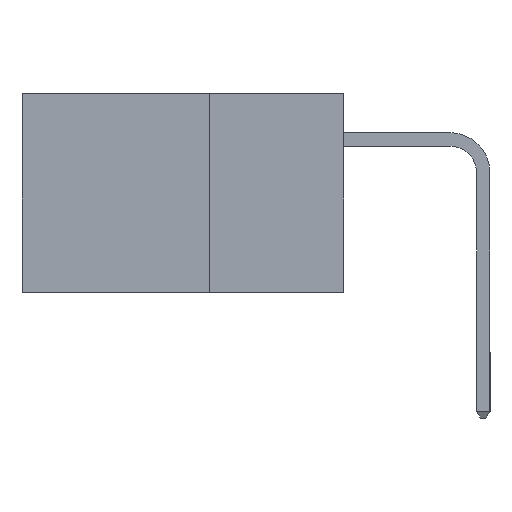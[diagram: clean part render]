
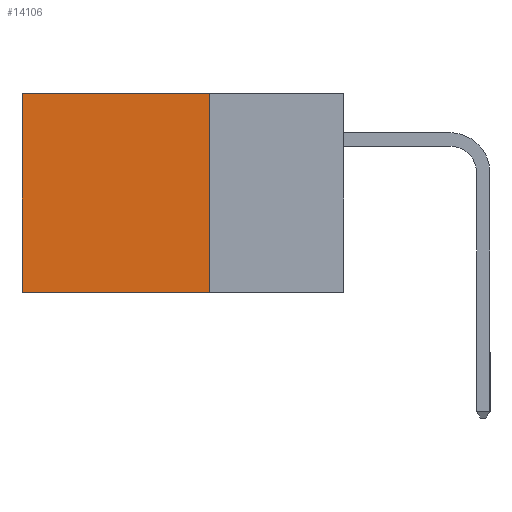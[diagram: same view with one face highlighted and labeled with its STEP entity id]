
A CAD part, left-side view. The second image highlights one B-rep face of the part: STEP entity #14106.
In plain terms, the highlighted planar face has unit normal (-1, 0, 0).
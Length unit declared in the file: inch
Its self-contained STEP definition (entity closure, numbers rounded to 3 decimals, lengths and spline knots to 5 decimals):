
#1137 = VERTEX_POINT ( 'NONE', #16307 ) ;
#2282 = ORIENTED_EDGE ( 'NONE', *, *, #13329, .F. ) ;
#2816 = EDGE_CURVE ( 'NONE', #12276, #1137, #12983, .T. ) ;
#3709 = CARTESIAN_POINT ( 'NONE',  ( 0.298, 0.25, 0. ) ) ;
#4359 = DIRECTION ( 'NONE',  ( 1., 0., 0. ) ) ;
#6640 = DIRECTION ( 'NONE',  ( 0., 0., -1. ) ) ;
#8068 = VERTEX_POINT ( 'NONE', #31557 ) ;
#9937 = VECTOR ( 'NONE', #20632, 39.37008 ) ;
#11472 = FACE_OUTER_BOUND ( 'NONE', #29227, .T. ) ;
#12276 = VERTEX_POINT ( 'NONE', #16536 ) ;
#12983 = LINE ( 'NONE', #14880, #30200 ) ;
#13329 = EDGE_CURVE ( 'NONE', #8068, #31857, #22819, .T. ) ;
#13431 = EDGE_CURVE ( 'NONE', #31857, #1137, #15075, .T. ) ;
#13539 = ORIENTED_EDGE ( 'NONE', *, *, #13992, .T. ) ;
#13589 = DIRECTION ( 'NONE',  ( 0., 1., 0. ) ) ;
#13992 = EDGE_CURVE ( 'NONE', #8068, #12276, #14637, .T. ) ;
#14106 = ADVANCED_FACE ( 'NONE', ( #11472 ), #29112, .F. ) ;
#14460 = DIRECTION ( 'NONE',  ( 0., 0., -1. ) ) ;
#14466 = ORIENTED_EDGE ( 'NONE', *, *, #13431, .F. ) ;
#14637 = LINE ( 'NONE', #3709, #20111 ) ;
#14880 = CARTESIAN_POINT ( 'NONE',  ( 0.298, 0.6, 0. ) ) ;
#15075 = LINE ( 'NONE', #20850, #9937 ) ;
#16307 = CARTESIAN_POINT ( 'NONE',  ( 0.298, 0.6, -0.37 ) ) ;
#16536 = CARTESIAN_POINT ( 'NONE',  ( 0.298, 0.6, 0. ) ) ;
#16761 = ORIENTED_EDGE ( 'NONE', *, *, #2816, .T. ) ;
#20111 = VECTOR ( 'NONE', #13589, 39.37008 ) ;
#20632 = DIRECTION ( 'NONE',  ( 0., 1., 0. ) ) ;
#20850 = CARTESIAN_POINT ( 'NONE',  ( 0.298, 0.25, -0.37 ) ) ;
#22819 = LINE ( 'NONE', #30141, #31864 ) ;
#24394 = CARTESIAN_POINT ( 'NONE',  ( 0.298, 0.25, 0. ) ) ;
#24871 = DIRECTION ( 'NONE',  ( 0., 0., -1. ) ) ;
#25568 = AXIS2_PLACEMENT_3D ( 'NONE', #24394, #4359, #14460 ) ;
#27161 = CARTESIAN_POINT ( 'NONE',  ( 0.298, 0.25, -0.37 ) ) ;
#29112 = PLANE ( 'NONE',  #25568 ) ;
#29227 = EDGE_LOOP ( 'NONE', ( #16761, #14466, #2282, #13539 ) ) ;
#30141 = CARTESIAN_POINT ( 'NONE',  ( 0.298, 0.25, 0. ) ) ;
#30200 = VECTOR ( 'NONE', #6640, 39.37008 ) ;
#31557 = CARTESIAN_POINT ( 'NONE',  ( 0.298, 0.25, 0. ) ) ;
#31857 = VERTEX_POINT ( 'NONE', #27161 ) ;
#31864 = VECTOR ( 'NONE', #24871, 39.37008 ) ;
